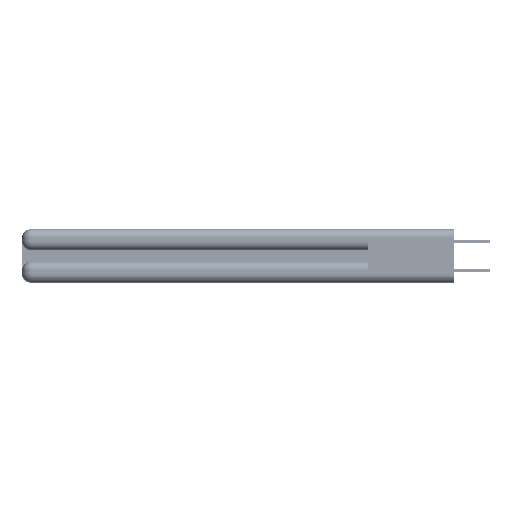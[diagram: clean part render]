
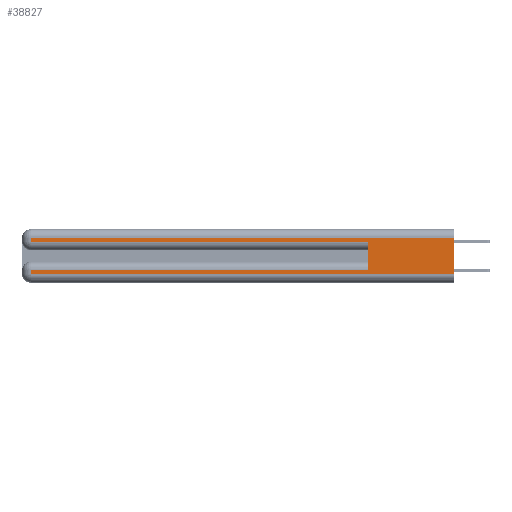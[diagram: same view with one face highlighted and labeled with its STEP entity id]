
A CAD part, left-side view. The second image highlights one B-rep face of the part: STEP entity #38827.
In plain terms, the highlighted planar face has unit normal (-1, 0, 0).
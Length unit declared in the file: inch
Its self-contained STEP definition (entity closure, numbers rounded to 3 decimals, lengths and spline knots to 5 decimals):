
#320 = LINE ( 'NONE', #20381, #22552 ) ;
#1310 = ORIENTED_EDGE ( 'NONE', *, *, #4966, .F. ) ;
#1313 = EDGE_CURVE ( 'NONE', #26393, #35881, #34117, .T. ) ;
#4472 = LINE ( 'NONE', #11946, #49570 ) ;
#4966 = EDGE_CURVE ( 'NONE', #37370, #14186, #320, .T. ) ;
#5274 = VECTOR ( 'NONE', #16344, 39.37008 ) ;
#6262 = ORIENTED_EDGE ( 'NONE', *, *, #50819, .T. ) ;
#6626 = DIRECTION ( 'NONE',  ( 0., 0., -1. ) ) ;
#7002 = VECTOR ( 'NONE', #39574, 39.37008 ) ;
#9551 = ORIENTED_EDGE ( 'NONE', *, *, #11178, .F. ) ;
#11024 = ORIENTED_EDGE ( 'NONE', *, *, #39157, .T. ) ;
#11170 = ORIENTED_EDGE ( 'NONE', *, *, #33215, .T. ) ;
#11178 = EDGE_CURVE ( 'NONE', #23679, #35881, #4472, .T. ) ;
#11735 = CARTESIAN_POINT ( 'NONE',  ( 0., 0., 0.085 ) ) ;
#11946 = CARTESIAN_POINT ( 'NONE',  ( 0., 0.6, 0.145 ) ) ;
#12418 = CARTESIAN_POINT ( 'NONE',  ( 0., 0., 0.285 ) ) ;
#12759 = DIRECTION ( 'NONE',  ( 0., 0., -1. ) ) ;
#13085 = VERTEX_POINT ( 'NONE', #28233 ) ;
#14186 = VERTEX_POINT ( 'NONE', #39697 ) ;
#15742 = CARTESIAN_POINT ( 'NONE',  ( 0., 0., 0.37 ) ) ;
#15840 = LINE ( 'NONE', #11735, #41883 ) ;
#16344 = DIRECTION ( 'NONE',  ( 0., -1., 0. ) ) ;
#16806 = DIRECTION ( 'NONE',  ( 0., 0., -1. ) ) ;
#17347 = AXIS2_PLACEMENT_3D ( 'NONE', #15742, #27352, #16806 ) ;
#17450 = EDGE_CURVE ( 'NONE', #23679, #46563, #15840, .T. ) ;
#19398 = EDGE_LOOP ( 'NONE', ( #1310, #11170, #11024, #28166, #9551, #31359, #20393, #6262 ) ) ;
#20381 = CARTESIAN_POINT ( 'NONE',  ( 0., 0., 0.37 ) ) ;
#20393 = ORIENTED_EDGE ( 'NONE', *, *, #46617, .T. ) ;
#21726 = LINE ( 'NONE', #31200, #40265 ) ;
#21912 = CARTESIAN_POINT ( 'NONE',  ( 0., 0.6, 0.285 ) ) ;
#22533 = CARTESIAN_POINT ( 'NONE',  ( 0., 0.6, 0.085 ) ) ;
#22552 = VECTOR ( 'NONE', #12759, 39.37008 ) ;
#23679 = VERTEX_POINT ( 'NONE', #22533 ) ;
#26393 = VERTEX_POINT ( 'NONE', #34668 ) ;
#27352 = DIRECTION ( 'NONE',  ( 1., 0., 0. ) ) ;
#28166 = ORIENTED_EDGE ( 'NONE', *, *, #1313, .T. ) ;
#28233 = CARTESIAN_POINT ( 'NONE',  ( 0., 2.94, 0.31 ) ) ;
#28518 = DIRECTION ( 'NONE',  ( 0., -1., 0. ) ) ;
#29545 = LINE ( 'NONE', #46019, #38847 ) ;
#31200 = CARTESIAN_POINT ( 'NONE',  ( 0., 2.94, 0.37 ) ) ;
#31359 = ORIENTED_EDGE ( 'NONE', *, *, #17450, .T. ) ;
#32299 = LINE ( 'NONE', #43710, #7002 ) ;
#32352 = DIRECTION ( 'NONE',  ( 0., 0., 1. ) ) ;
#32407 = LINE ( 'NONE', #44197, #5274 ) ;
#33215 = EDGE_CURVE ( 'NONE', #37370, #13085, #32299, .T. ) ;
#34117 = LINE ( 'NONE', #12418, #45861 ) ;
#34668 = CARTESIAN_POINT ( 'NONE',  ( 0., 2.94, 0.285 ) ) ;
#35117 = CARTESIAN_POINT ( 'NONE',  ( 0., 0., 0.31 ) ) ;
#35187 = FACE_OUTER_BOUND ( 'NONE', #19398, .T. ) ;
#35881 = VERTEX_POINT ( 'NONE', #21912 ) ;
#37370 = VERTEX_POINT ( 'NONE', #35117 ) ;
#38827 = ADVANCED_FACE ( 'NONE', ( #35187 ), #50989, .F. ) ;
#38847 = VECTOR ( 'NONE', #6626, 39.37008 ) ;
#39157 = EDGE_CURVE ( 'NONE', #13085, #26393, #29545, .T. ) ;
#39574 = DIRECTION ( 'NONE',  ( 0., 1., 0. ) ) ;
#39697 = CARTESIAN_POINT ( 'NONE',  ( 0., 0., 0.06 ) ) ;
#40265 = VECTOR ( 'NONE', #43140, 39.37008 ) ;
#40422 = VERTEX_POINT ( 'NONE', #48681 ) ;
#41883 = VECTOR ( 'NONE', #47691, 39.37008 ) ;
#43140 = DIRECTION ( 'NONE',  ( 0., 0., -1. ) ) ;
#43311 = CARTESIAN_POINT ( 'NONE',  ( 0., 2.94, 0.085 ) ) ;
#43710 = CARTESIAN_POINT ( 'NONE',  ( 0., 0., 0.31 ) ) ;
#44197 = CARTESIAN_POINT ( 'NONE',  ( 0., 0., 0.06 ) ) ;
#45861 = VECTOR ( 'NONE', #28518, 39.37008 ) ;
#46019 = CARTESIAN_POINT ( 'NONE',  ( 0., 2.94, 0.37 ) ) ;
#46563 = VERTEX_POINT ( 'NONE', #43311 ) ;
#46617 = EDGE_CURVE ( 'NONE', #46563, #40422, #21726, .T. ) ;
#47691 = DIRECTION ( 'NONE',  ( 0., 1., 0. ) ) ;
#48681 = CARTESIAN_POINT ( 'NONE',  ( 0., 2.94, 0.06 ) ) ;
#49570 = VECTOR ( 'NONE', #32352, 39.37008 ) ;
#50819 = EDGE_CURVE ( 'NONE', #40422, #14186, #32407, .T. ) ;
#50989 = PLANE ( 'NONE',  #17347 ) ;
